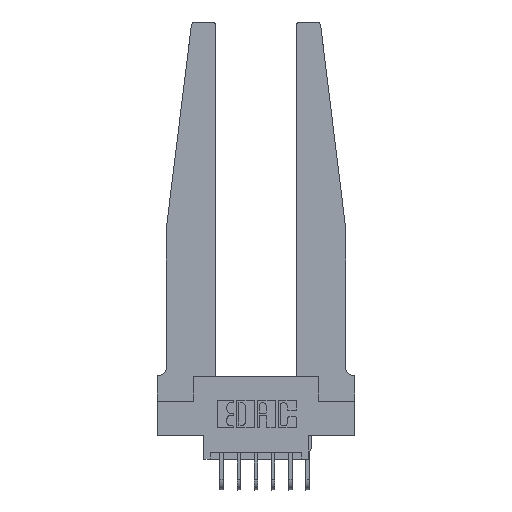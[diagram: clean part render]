
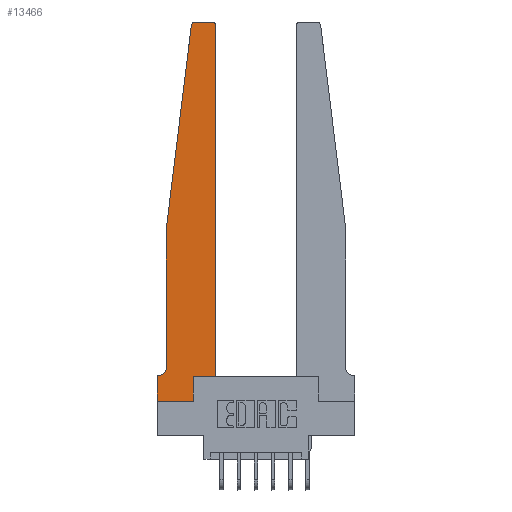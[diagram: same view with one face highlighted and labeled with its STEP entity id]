
A CAD part, top view. The second image highlights one B-rep face of the part: STEP entity #13466.
In plain terms, the highlighted planar face has unit normal (0, 0, 1).
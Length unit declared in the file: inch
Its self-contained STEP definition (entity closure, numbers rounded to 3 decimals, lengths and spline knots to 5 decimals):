
#21 = LINE ( 'NONE', #13044, #3219 ) ;
#536 = EDGE_CURVE ( 'NONE', #7210, #4127, #6112, .T. ) ;
#723 = ORIENTED_EDGE ( 'NONE', *, *, #7524, .T. ) ;
#837 = EDGE_CURVE ( 'NONE', #8554, #5337, #2420, .T. ) ;
#958 = CARTESIAN_POINT ( 'NONE',  ( 0.015, 0.1875, 0.37 ) ) ;
#1114 = ORIENTED_EDGE ( 'NONE', *, *, #12272, .T. ) ;
#1301 = ORIENTED_EDGE ( 'NONE', *, *, #4211, .T. ) ;
#1302 = CARTESIAN_POINT ( 'NONE',  ( 0.065, 0.2375, 0.37 ) ) ;
#1319 = CARTESIAN_POINT ( 'NONE',  ( 0.2605, 0.18, 0.37 ) ) ;
#1675 = LINE ( 'NONE', #5401, #10255 ) ;
#1842 = EDGE_CURVE ( 'NONE', #4540, #7529, #5949, .T. ) ;
#2025 = ORIENTED_EDGE ( 'NONE', *, *, #837, .T. ) ;
#2038 = EDGE_CURVE ( 'NONE', #5337, #7210, #11985, .T. ) ;
#2054 = ORIENTED_EDGE ( 'NONE', *, *, #2038, .T. ) ;
#2298 = AXIS2_PLACEMENT_3D ( 'NONE', #10699, #9623, #5083 ) ;
#2326 = DIRECTION ( 'NONE',  ( 0., 0., -1. ) ) ;
#2420 = CIRCLE ( 'NONE', #12092, 0.03 ) ;
#2622 = ORIENTED_EDGE ( 'NONE', *, *, #9113, .T. ) ;
#2726 = CARTESIAN_POINT ( 'NONE',  ( 0.065, 1.25, 0.37 ) ) ;
#3192 = ORIENTED_EDGE ( 'NONE', *, *, #536, .T. ) ;
#3219 = VECTOR ( 'NONE', #3688, 39.37008 ) ;
#3396 = DIRECTION ( 'NONE',  ( -1., 0., 0. ) ) ;
#3688 = DIRECTION ( 'NONE',  ( 0., 1., 0. ) ) ;
#3861 = ORIENTED_EDGE ( 'NONE', *, *, #1842, .T. ) ;
#3988 = AXIS2_PLACEMENT_3D ( 'NONE', #8248, #2326, #11836 ) ;
#4127 = VERTEX_POINT ( 'NONE', #1302 ) ;
#4211 = EDGE_CURVE ( 'NONE', #13935, #8539, #14734, .T. ) ;
#4540 = VERTEX_POINT ( 'NONE', #12114 ) ;
#4567 = VECTOR ( 'NONE', #3396, 39.37008 ) ;
#4839 = CARTESIAN_POINT ( 'NONE',  ( 0.065, 1.25, 0.37 ) ) ;
#5057 = CARTESIAN_POINT ( 'NONE',  ( 0., 0.1875, 0.37 ) ) ;
#5083 = DIRECTION ( 'NONE',  ( 1., 0., 0. ) ) ;
#5225 = DIRECTION ( 'NONE',  ( 0., -1., 0. ) ) ;
#5245 = DIRECTION ( 'NONE',  ( 1., 0., 0. ) ) ;
#5337 = VERTEX_POINT ( 'NONE', #12376 ) ;
#5340 = EDGE_LOOP ( 'NONE', ( #723, #2025, #2054, #3192, #11583, #2622, #15387, #7067, #1301, #1114, #13684, #3861 ) ) ;
#5401 = CARTESIAN_POINT ( 'NONE',  ( 0.425, 0.18, 0.37 ) ) ;
#5406 = EDGE_CURVE ( 'NONE', #13240, #13935, #12136, .T. ) ;
#5567 = VERTEX_POINT ( 'NONE', #6684 ) ;
#5774 = VECTOR ( 'NONE', #10911, 39.37008 ) ;
#5949 = CIRCLE ( 'NONE', #14670, 0.03 ) ;
#6112 = LINE ( 'NONE', #2726, #9352 ) ;
#6683 = DIRECTION ( 'NONE',  ( 0., -1., 0. ) ) ;
#6684 = CARTESIAN_POINT ( 'NONE',  ( 0.425, 0.18, 0.37 ) ) ;
#6845 = CARTESIAN_POINT ( 'NONE',  ( 0.395, 2.75, 0.37 ) ) ;
#6915 = LINE ( 'NONE', #8019, #4567 ) ;
#7067 = ORIENTED_EDGE ( 'NONE', *, *, #5406, .T. ) ;
#7210 = VERTEX_POINT ( 'NONE', #4839 ) ;
#7265 = FACE_OUTER_BOUND ( 'NONE', #5340, .T. ) ;
#7315 = CARTESIAN_POINT ( 'NONE',  ( 0.2605, 0.18, 0.37 ) ) ;
#7494 = CARTESIAN_POINT ( 'NONE',  ( 0.395, 2.72, 0.37 ) ) ;
#7524 = EDGE_CURVE ( 'NONE', #7529, #8554, #6915, .T. ) ;
#7529 = VERTEX_POINT ( 'NONE', #6845 ) ;
#7878 = VECTOR ( 'NONE', #12517, 39.37008 ) ;
#8019 = CARTESIAN_POINT ( 'NONE',  ( 0.25, 2.75, 0.37 ) ) ;
#8248 = CARTESIAN_POINT ( 'NONE',  ( 0.015, 0.2375, 0.37 ) ) ;
#8250 = CARTESIAN_POINT ( 'NONE',  ( 0.065, 1.25, 0.37 ) ) ;
#8539 = VERTEX_POINT ( 'NONE', #1319 ) ;
#8554 = VERTEX_POINT ( 'NONE', #9844 ) ;
#9113 = EDGE_CURVE ( 'NONE', #9641, #12943, #12433, .T. ) ;
#9206 = DIRECTION ( 'NONE',  ( 0., 0., 1. ) ) ;
#9352 = VECTOR ( 'NONE', #5225, 39.37008 ) ;
#9623 = DIRECTION ( 'NONE',  ( 0., 0., 1. ) ) ;
#9641 = VERTEX_POINT ( 'NONE', #958 ) ;
#9652 = CARTESIAN_POINT ( 'NONE',  ( 0.27653, 2.72, 0.37 ) ) ;
#9844 = CARTESIAN_POINT ( 'NONE',  ( 0.27653, 2.75, 0.37 ) ) ;
#10204 = CARTESIAN_POINT ( 'NONE',  ( 0., 0., 0.37 ) ) ;
#10255 = VECTOR ( 'NONE', #5245, 39.37008 ) ;
#10268 = VECTOR ( 'NONE', #14589, 39.37008 ) ;
#10451 = DIRECTION ( 'NONE',  ( 1., 0., 0. ) ) ;
#10699 = CARTESIAN_POINT ( 'NONE',  ( 0., 0.1875, 0.37 ) ) ;
#10718 = CIRCLE ( 'NONE', #3988, 0.05 ) ;
#10759 = EDGE_CURVE ( 'NONE', #5567, #4540, #21, .T. ) ;
#10895 = DIRECTION ( 'NONE',  ( 1., 0., 0. ) ) ;
#10911 = DIRECTION ( 'NONE',  ( 0., 1., 0. ) ) ;
#11140 = EDGE_CURVE ( 'NONE', #4127, #9641, #10718, .T. ) ;
#11333 = EDGE_CURVE ( 'NONE', #12943, #13240, #11376, .T. ) ;
#11376 = LINE ( 'NONE', #10204, #11955 ) ;
#11583 = ORIENTED_EDGE ( 'NONE', *, *, #11140, .T. ) ;
#11836 = DIRECTION ( 'NONE',  ( -1., 0., 0. ) ) ;
#11955 = VECTOR ( 'NONE', #6683, 39.37008 ) ;
#11985 = LINE ( 'NONE', #8250, #13932 ) ;
#12092 = AXIS2_PLACEMENT_3D ( 'NONE', #9652, #14403, #10895 ) ;
#12112 = CARTESIAN_POINT ( 'NONE',  ( 0.2605, 0., 0.37 ) ) ;
#12114 = CARTESIAN_POINT ( 'NONE',  ( 0.425, 2.72, 0.37 ) ) ;
#12136 = LINE ( 'NONE', #14819, #10268 ) ;
#12272 = EDGE_CURVE ( 'NONE', #8539, #5567, #1675, .T. ) ;
#12376 = CARTESIAN_POINT ( 'NONE',  ( 0.24675, 2.72367, 0.37 ) ) ;
#12433 = LINE ( 'NONE', #13467, #7878 ) ;
#12517 = DIRECTION ( 'NONE',  ( -1., 0., 0. ) ) ;
#12581 = CARTESIAN_POINT ( 'NONE',  ( 0., 0., 0.37 ) ) ;
#12943 = VERTEX_POINT ( 'NONE', #5057 ) ;
#13044 = CARTESIAN_POINT ( 'NONE',  ( 0.425, 0.18, 0.37 ) ) ;
#13240 = VERTEX_POINT ( 'NONE', #12581 ) ;
#13263 = PLANE ( 'NONE',  #2298 ) ;
#13466 = ADVANCED_FACE ( 'NONE', ( #7265 ), #13263, .T. ) ;
#13467 = CARTESIAN_POINT ( 'NONE',  ( 0.065, 0.1875, 0.37 ) ) ;
#13684 = ORIENTED_EDGE ( 'NONE', *, *, #10759, .T. ) ;
#13932 = VECTOR ( 'NONE', #14352, 39.37008 ) ;
#13935 = VERTEX_POINT ( 'NONE', #12112 ) ;
#14352 = DIRECTION ( 'NONE',  ( -0.122, -0.992, 0. ) ) ;
#14403 = DIRECTION ( 'NONE',  ( 0., 0., 1. ) ) ;
#14589 = DIRECTION ( 'NONE',  ( 1., 0., 0. ) ) ;
#14670 = AXIS2_PLACEMENT_3D ( 'NONE', #7494, #9206, #10451 ) ;
#14734 = LINE ( 'NONE', #7315, #5774 ) ;
#14819 = CARTESIAN_POINT ( 'NONE',  ( 0., 0., 0.37 ) ) ;
#15387 = ORIENTED_EDGE ( 'NONE', *, *, #11333, .T. ) ;
